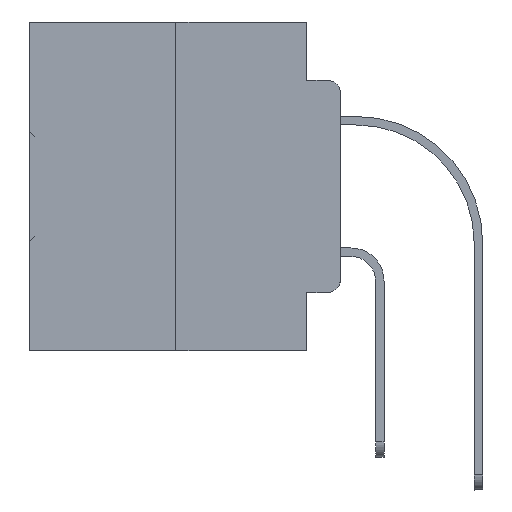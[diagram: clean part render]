
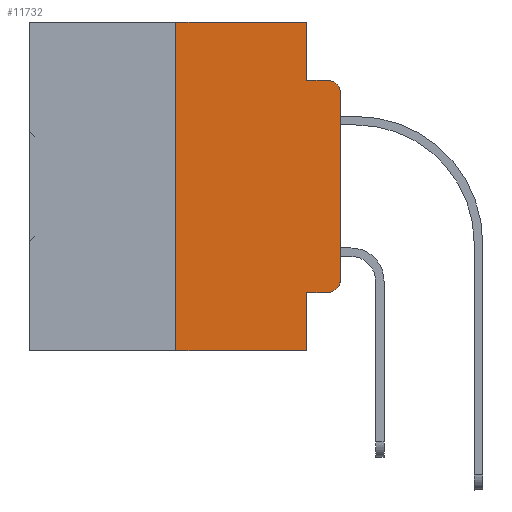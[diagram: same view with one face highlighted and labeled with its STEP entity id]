
A CAD part, left-side view. The second image highlights one B-rep face of the part: STEP entity #11732.
In plain terms, the highlighted planar face has unit normal (-1, 0, 0).
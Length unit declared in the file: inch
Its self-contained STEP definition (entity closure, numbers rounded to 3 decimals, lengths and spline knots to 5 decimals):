
#301 = AXIS2_PLACEMENT_3D ( 'NONE', #4156, #3968, #10086 ) ;
#748 = CARTESIAN_POINT ( 'NONE',  ( 0., 0.051, -0.4115 ) ) ;
#840 = VECTOR ( 'NONE', #10222, 39.37008 ) ;
#1383 = ORIENTED_EDGE ( 'NONE', *, *, #19975, .F. ) ;
#1895 = ORIENTED_EDGE ( 'NONE', *, *, #9585, .F. ) ;
#2001 = LINE ( 'NONE', #24749, #37497 ) ;
#2700 = CARTESIAN_POINT ( 'NONE',  ( 0., 0.051, -0.4115 ) ) ;
#2877 = CARTESIAN_POINT ( 'NONE',  ( 0., 0., -0.1085 ) ) ;
#2928 = LINE ( 'NONE', #32517, #15464 ) ;
#3495 = DIRECTION ( 'NONE',  ( 0., 0., 1. ) ) ;
#3868 = EDGE_CURVE ( 'NONE', #32865, #31354, #2928, .T. ) ;
#3968 = DIRECTION ( 'NONE',  ( -1., 0., 0. ) ) ;
#4034 = PLANE ( 'NONE',  #11382 ) ;
#4156 = CARTESIAN_POINT ( 'NONE',  ( 0., 0.02, -0.3915 ) ) ;
#4492 = CARTESIAN_POINT ( 'NONE',  ( 0., 0.051, 0. ) ) ;
#4559 = CIRCLE ( 'NONE', #6401, 0.02 ) ;
#5267 = VECTOR ( 'NONE', #6369, 39.37008 ) ;
#5269 = EDGE_CURVE ( 'NONE', #35606, #9941, #10200, .T. ) ;
#5554 = VERTEX_POINT ( 'NONE', #2700 ) ;
#6369 = DIRECTION ( 'NONE',  ( 0., -1., 0. ) ) ;
#6401 = AXIS2_PLACEMENT_3D ( 'NONE', #14136, #34897, #22544 ) ;
#6909 = FACE_OUTER_BOUND ( 'NONE', #27442, .T. ) ;
#7294 = VECTOR ( 'NONE', #32350, 39.37008 ) ;
#7612 = CARTESIAN_POINT ( 'NONE',  ( 0., 0.051, 0. ) ) ;
#8512 = VECTOR ( 'NONE', #24449, 39.37008 ) ;
#9268 = CARTESIAN_POINT ( 'NONE',  ( 0., 0.051, -0.5 ) ) ;
#9585 = EDGE_CURVE ( 'NONE', #9941, #25745, #33762, .T. ) ;
#9941 = VERTEX_POINT ( 'NONE', #36506 ) ;
#10083 = ORIENTED_EDGE ( 'NONE', *, *, #5269, .F. ) ;
#10086 = DIRECTION ( 'NONE',  ( 0., 0., -1. ) ) ;
#10200 = LINE ( 'NONE', #24702, #35978 ) ;
#10222 = DIRECTION ( 'NONE',  ( 0., 0., -1. ) ) ;
#10802 = EDGE_CURVE ( 'NONE', #15791, #35537, #2001, .T. ) ;
#11382 = AXIS2_PLACEMENT_3D ( 'NONE', #15699, #12837, #33233 ) ;
#11471 = ORIENTED_EDGE ( 'NONE', *, *, #19365, .T. ) ;
#11732 = ADVANCED_FACE ( 'NONE', ( #6909 ), #4034, .F. ) ;
#12609 = LINE ( 'NONE', #748, #8512 ) ;
#12837 = DIRECTION ( 'NONE',  ( 1., 0., 0. ) ) ;
#12989 = ORIENTED_EDGE ( 'NONE', *, *, #10802, .T. ) ;
#13738 = CARTESIAN_POINT ( 'NONE',  ( 0., 0.051, -0.0885 ) ) ;
#14136 = CARTESIAN_POINT ( 'NONE',  ( 0., 0.02, -0.1085 ) ) ;
#15296 = ORIENTED_EDGE ( 'NONE', *, *, #36198, .T. ) ;
#15464 = VECTOR ( 'NONE', #3495, 39.37008 ) ;
#15699 = CARTESIAN_POINT ( 'NONE',  ( 0., 0.473, 0. ) ) ;
#15791 = VERTEX_POINT ( 'NONE', #37013 ) ;
#17168 = ORIENTED_EDGE ( 'NONE', *, *, #30566, .F. ) ;
#18411 = EDGE_CURVE ( 'NONE', #5554, #35537, #30635, .T. ) ;
#18957 = EDGE_CURVE ( 'NONE', #31354, #28212, #4559, .T. ) ;
#19035 = VERTEX_POINT ( 'NONE', #23094 ) ;
#19365 = EDGE_CURVE ( 'NONE', #19035, #32865, #28369, .T. ) ;
#19975 = EDGE_CURVE ( 'NONE', #25745, #28212, #32515, .T. ) ;
#21167 = CARTESIAN_POINT ( 'NONE',  ( 0., 0.02, -0.0885 ) ) ;
#21889 = DIRECTION ( 'NONE',  ( 0., -1., 0. ) ) ;
#22544 = DIRECTION ( 'NONE',  ( 0., 0., -1. ) ) ;
#22710 = DIRECTION ( 'NONE',  ( 0., 0., -1. ) ) ;
#23094 = CARTESIAN_POINT ( 'NONE',  ( 0., 0.02, -0.4115 ) ) ;
#23566 = ORIENTED_EDGE ( 'NONE', *, *, #18957, .T. ) ;
#24449 = DIRECTION ( 'NONE',  ( 0., -1., 0. ) ) ;
#24655 = CARTESIAN_POINT ( 'NONE',  ( 0., 0., -0.3915 ) ) ;
#24702 = CARTESIAN_POINT ( 'NONE',  ( 0., 0.473, 0. ) ) ;
#24749 = CARTESIAN_POINT ( 'NONE',  ( 0., 0.473, -0.5 ) ) ;
#25621 = ORIENTED_EDGE ( 'NONE', *, *, #18411, .F. ) ;
#25745 = VERTEX_POINT ( 'NONE', #13738 ) ;
#26239 = CARTESIAN_POINT ( 'NONE',  ( 0., 0.051, -0.0885 ) ) ;
#27182 = DIRECTION ( 'NONE',  ( 0., -1., 0. ) ) ;
#27204 = CARTESIAN_POINT ( 'NONE',  ( 0., 0.25, 0. ) ) ;
#27442 = EDGE_LOOP ( 'NONE', ( #30045, #23566, #1383, #1895, #10083, #17168, #12989, #25621, #15296, #11471 ) ) ;
#28212 = VERTEX_POINT ( 'NONE', #21167 ) ;
#28369 = CIRCLE ( 'NONE', #301, 0.02 ) ;
#29095 = CARTESIAN_POINT ( 'NONE',  ( 0., 0.25, 0. ) ) ;
#30045 = ORIENTED_EDGE ( 'NONE', *, *, #3868, .T. ) ;
#30566 = EDGE_CURVE ( 'NONE', #15791, #35606, #32150, .T. ) ;
#30635 = LINE ( 'NONE', #4492, #840 ) ;
#31354 = VERTEX_POINT ( 'NONE', #2877 ) ;
#32150 = LINE ( 'NONE', #29095, #7294 ) ;
#32350 = DIRECTION ( 'NONE',  ( 0., 0., 1. ) ) ;
#32515 = LINE ( 'NONE', #26239, #5267 ) ;
#32517 = CARTESIAN_POINT ( 'NONE',  ( 0., 0., 0. ) ) ;
#32865 = VERTEX_POINT ( 'NONE', #24655 ) ;
#33233 = DIRECTION ( 'NONE',  ( 0., 0., -1. ) ) ;
#33762 = LINE ( 'NONE', #7612, #35541 ) ;
#34897 = DIRECTION ( 'NONE',  ( -1., 0., 0. ) ) ;
#35537 = VERTEX_POINT ( 'NONE', #9268 ) ;
#35541 = VECTOR ( 'NONE', #22710, 39.37008 ) ;
#35606 = VERTEX_POINT ( 'NONE', #27204 ) ;
#35978 = VECTOR ( 'NONE', #27182, 39.37008 ) ;
#36198 = EDGE_CURVE ( 'NONE', #5554, #19035, #12609, .T. ) ;
#36506 = CARTESIAN_POINT ( 'NONE',  ( 0., 0.051, 0. ) ) ;
#37013 = CARTESIAN_POINT ( 'NONE',  ( 0., 0.25, -0.5 ) ) ;
#37497 = VECTOR ( 'NONE', #21889, 39.37008 ) ;
